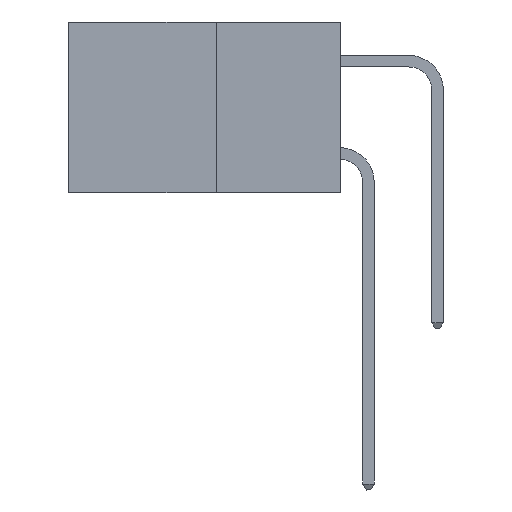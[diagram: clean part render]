
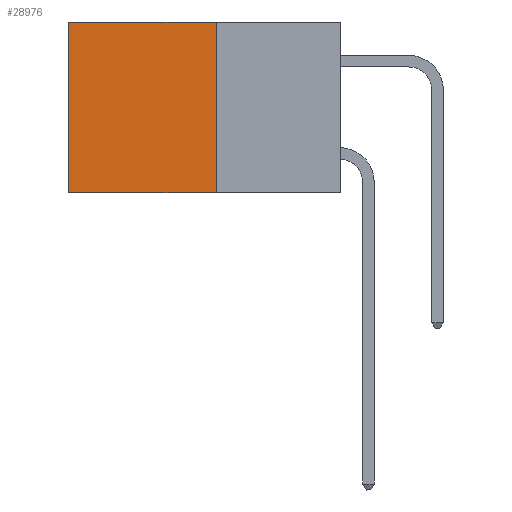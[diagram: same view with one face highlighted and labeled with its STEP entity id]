
A CAD part, left-side view. The second image highlights one B-rep face of the part: STEP entity #28976.
In plain terms, the highlighted planar face has unit normal (-1, 0, 0).
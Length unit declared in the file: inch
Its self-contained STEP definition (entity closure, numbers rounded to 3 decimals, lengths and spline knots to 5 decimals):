
#1270 = DIRECTION ( 'NONE',  ( 0., 0., -1. ) ) ;
#1948 = DIRECTION ( 'NONE',  ( 1., 0., 0. ) ) ;
#2961 = EDGE_LOOP ( 'NONE', ( #4133, #22592, #31134, #15338 ) ) ;
#3147 = CARTESIAN_POINT ( 'NONE',  ( 0.277, 0.27, -0.37 ) ) ;
#4133 = ORIENTED_EDGE ( 'NONE', *, *, #16190, .T. ) ;
#5713 = CARTESIAN_POINT ( 'NONE',  ( 0.277, 0.27, -0.37 ) ) ;
#6040 = VECTOR ( 'NONE', #20022, 39.37008 ) ;
#6580 = DIRECTION ( 'NONE',  ( 0., 0., -1. ) ) ;
#8816 = VERTEX_POINT ( 'NONE', #22458 ) ;
#9475 = CARTESIAN_POINT ( 'NONE',  ( 0.277, 0.59, -0.37 ) ) ;
#13333 = VECTOR ( 'NONE', #6580, 39.37008 ) ;
#13919 = EDGE_CURVE ( 'NONE', #14982, #16801, #36553, .T. ) ;
#14982 = VERTEX_POINT ( 'NONE', #15415 ) ;
#15023 = VECTOR ( 'NONE', #28768, 39.37008 ) ;
#15338 = ORIENTED_EDGE ( 'NONE', *, *, #17469, .T. ) ;
#15415 = CARTESIAN_POINT ( 'NONE',  ( 0.277, 0.27, 0. ) ) ;
#15924 = LINE ( 'NONE', #25924, #15023 ) ;
#16190 = EDGE_CURVE ( 'NONE', #8816, #34075, #27662, .T. ) ;
#16801 = VERTEX_POINT ( 'NONE', #3147 ) ;
#17469 = EDGE_CURVE ( 'NONE', #14982, #8816, #15924, .T. ) ;
#20022 = DIRECTION ( 'NONE',  ( 0., 1., 0. ) ) ;
#21533 = VECTOR ( 'NONE', #1270, 39.37008 ) ;
#22039 = DIRECTION ( 'NONE',  ( 0., 0., -1. ) ) ;
#22458 = CARTESIAN_POINT ( 'NONE',  ( 0.277, 0.59, 0. ) ) ;
#22592 = ORIENTED_EDGE ( 'NONE', *, *, #25233, .F. ) ;
#25233 = EDGE_CURVE ( 'NONE', #16801, #34075, #36314, .T. ) ;
#25540 = FACE_OUTER_BOUND ( 'NONE', #2961, .T. ) ;
#25615 = AXIS2_PLACEMENT_3D ( 'NONE', #36109, #1948, #22039 ) ;
#25924 = CARTESIAN_POINT ( 'NONE',  ( 0.277, 0.27, 0. ) ) ;
#27123 = CARTESIAN_POINT ( 'NONE',  ( 0.277, 0.27, -0.37 ) ) ;
#27662 = LINE ( 'NONE', #9475, #13333 ) ;
#28768 = DIRECTION ( 'NONE',  ( 0., 1., 0. ) ) ;
#28976 = ADVANCED_FACE ( 'NONE', ( #25540 ), #30493, .F. ) ;
#30493 = PLANE ( 'NONE',  #25615 ) ;
#31134 = ORIENTED_EDGE ( 'NONE', *, *, #13919, .F. ) ;
#34075 = VERTEX_POINT ( 'NONE', #36402 ) ;
#36109 = CARTESIAN_POINT ( 'NONE',  ( 0.277, 0.27, -0.37 ) ) ;
#36314 = LINE ( 'NONE', #5713, #6040 ) ;
#36402 = CARTESIAN_POINT ( 'NONE',  ( 0.277, 0.59, -0.37 ) ) ;
#36553 = LINE ( 'NONE', #27123, #21533 ) ;
